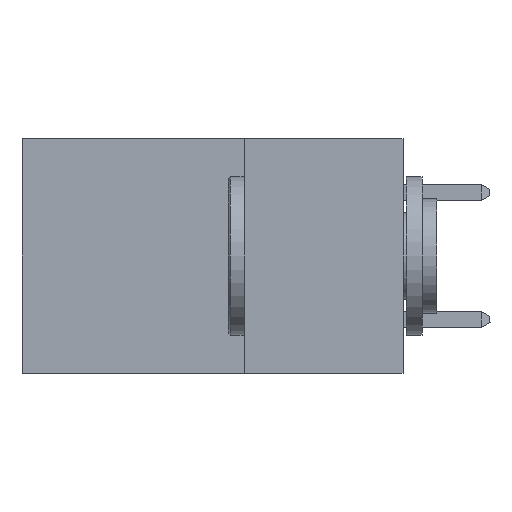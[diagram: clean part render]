
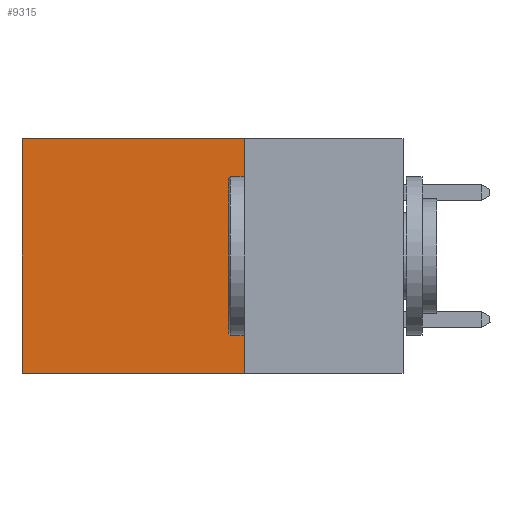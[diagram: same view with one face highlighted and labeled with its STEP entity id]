
A CAD part, left-side view. The second image highlights one B-rep face of the part: STEP entity #9315.
In plain terms, the highlighted planar face has unit normal (-1, 0, 0).
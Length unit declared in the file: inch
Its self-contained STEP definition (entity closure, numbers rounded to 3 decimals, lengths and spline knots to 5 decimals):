
#374 = EDGE_CURVE ( 'NONE', #4153, #10563, #6759, .T. ) ;
#580 = VECTOR ( 'NONE', #608, 39.37008 ) ;
#608 = DIRECTION ( 'NONE',  ( 0., 1., 0. ) ) ;
#1182 = CARTESIAN_POINT ( 'NONE',  ( 0.2875, 0.6, 0. ) ) ;
#1541 = CARTESIAN_POINT ( 'NONE',  ( 0.2875, 0.6, 0. ) ) ;
#1807 = DIRECTION ( 'NONE',  ( 0., 0., -1. ) ) ;
#3977 = ORIENTED_EDGE ( 'NONE', *, *, #374, .T. ) ;
#4153 = VERTEX_POINT ( 'NONE', #16190 ) ;
#5366 = EDGE_CURVE ( 'NONE', #4153, #13736, #15146, .T. ) ;
#5586 = ORIENTED_EDGE ( 'NONE', *, *, #11198, .T. ) ;
#6545 = PLANE ( 'NONE',  #19044 ) ;
#6759 = LINE ( 'NONE', #21572, #580 ) ;
#7571 = VECTOR ( 'NONE', #21797, 39.37008 ) ;
#7949 = EDGE_CURVE ( 'NONE', #13736, #11061, #8508, .T. ) ;
#8508 = LINE ( 'NONE', #9220, #19190 ) ;
#9220 = CARTESIAN_POINT ( 'NONE',  ( 0.2875, 0.25, -0.37 ) ) ;
#9315 = ADVANCED_FACE ( 'NONE', ( #17178 ), #6545, .F. ) ;
#10563 = VERTEX_POINT ( 'NONE', #1541 ) ;
#11061 = VERTEX_POINT ( 'NONE', #27074 ) ;
#11198 = EDGE_CURVE ( 'NONE', #10563, #11061, #13507, .T. ) ;
#12419 = VECTOR ( 'NONE', #21304, 39.37008 ) ;
#13507 = LINE ( 'NONE', #1182, #12419 ) ;
#13736 = VERTEX_POINT ( 'NONE', #22142 ) ;
#14792 = CARTESIAN_POINT ( 'NONE',  ( 0.2875, 0.25, 0. ) ) ;
#15146 = LINE ( 'NONE', #14792, #7571 ) ;
#15568 = CARTESIAN_POINT ( 'NONE',  ( 0.2875, 0.25, 0. ) ) ;
#15847 = ORIENTED_EDGE ( 'NONE', *, *, #7949, .F. ) ;
#16190 = CARTESIAN_POINT ( 'NONE',  ( 0.2875, 0.25, 0. ) ) ;
#17178 = FACE_OUTER_BOUND ( 'NONE', #24763, .T. ) ;
#19044 = AXIS2_PLACEMENT_3D ( 'NONE', #15568, #26792, #1807 ) ;
#19190 = VECTOR ( 'NONE', #27579, 39.37008 ) ;
#21304 = DIRECTION ( 'NONE',  ( 0., 0., -1. ) ) ;
#21572 = CARTESIAN_POINT ( 'NONE',  ( 0.2875, 0.25, 0. ) ) ;
#21797 = DIRECTION ( 'NONE',  ( 0., 0., -1. ) ) ;
#22142 = CARTESIAN_POINT ( 'NONE',  ( 0.2875, 0.25, -0.37 ) ) ;
#24763 = EDGE_LOOP ( 'NONE', ( #5586, #15847, #25285, #3977 ) ) ;
#25285 = ORIENTED_EDGE ( 'NONE', *, *, #5366, .F. ) ;
#26792 = DIRECTION ( 'NONE',  ( 1., 0., 0. ) ) ;
#27074 = CARTESIAN_POINT ( 'NONE',  ( 0.2875, 0.6, -0.37 ) ) ;
#27579 = DIRECTION ( 'NONE',  ( 0., 1., 0. ) ) ;
